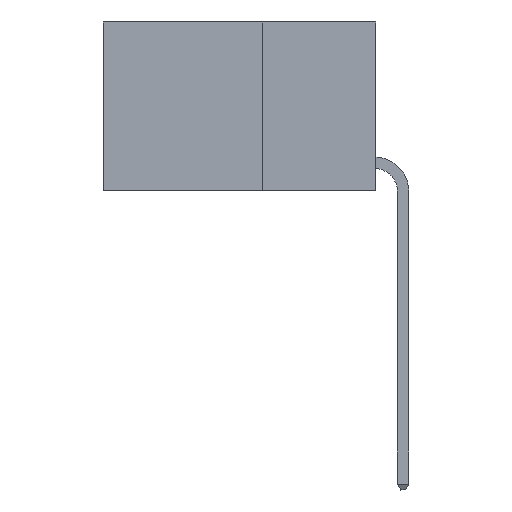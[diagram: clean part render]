
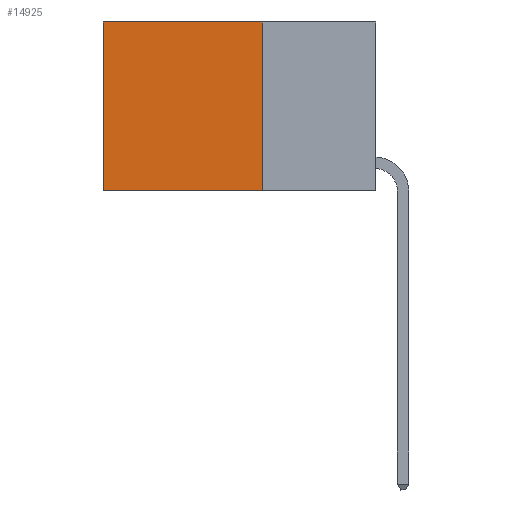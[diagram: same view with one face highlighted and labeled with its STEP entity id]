
A CAD part, left-side view. The second image highlights one B-rep face of the part: STEP entity #14925.
In plain terms, the highlighted planar face has unit normal (-1, 0, 0).
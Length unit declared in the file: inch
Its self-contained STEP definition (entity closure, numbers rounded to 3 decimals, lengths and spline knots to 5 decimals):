
#178 = EDGE_LOOP ( 'NONE', ( #12319, #1193, #4181, #5800 ) ) ;
#631 = FACE_OUTER_BOUND ( 'NONE', #178, .T. ) ;
#1193 = ORIENTED_EDGE ( 'NONE', *, *, #12555, .F. ) ;
#1260 = DIRECTION ( 'NONE',  ( 0., 0., -1. ) ) ;
#2142 = DIRECTION ( 'NONE',  ( 0., 1., 0. ) ) ;
#2449 = LINE ( 'NONE', #5815, #4506 ) ;
#2933 = VECTOR ( 'NONE', #1260, 39.37008 ) ;
#3328 = LINE ( 'NONE', #11789, #2933 ) ;
#3760 = DIRECTION ( 'NONE',  ( 0., 0., -1. ) ) ;
#4181 = ORIENTED_EDGE ( 'NONE', *, *, #6781, .F. ) ;
#4430 = EDGE_CURVE ( 'NONE', #8586, #11255, #3328, .T. ) ;
#4506 = VECTOR ( 'NONE', #7686, 39.37008 ) ;
#4978 = VERTEX_POINT ( 'NONE', #14207 ) ;
#5800 = ORIENTED_EDGE ( 'NONE', *, *, #12618, .T. ) ;
#5815 = CARTESIAN_POINT ( 'NONE',  ( 0.2625, 0.25, 0. ) ) ;
#5993 = CARTESIAN_POINT ( 'NONE',  ( 0.2625, 0.6, -0.37 ) ) ;
#6781 = EDGE_CURVE ( 'NONE', #4978, #9241, #12903, .T. ) ;
#6822 = CARTESIAN_POINT ( 'NONE',  ( 0.2625, 0.25, 0. ) ) ;
#7686 = DIRECTION ( 'NONE',  ( 0., 1., 0. ) ) ;
#7951 = DIRECTION ( 'NONE',  ( 0., 0., -1. ) ) ;
#8586 = VERTEX_POINT ( 'NONE', #13380 ) ;
#9241 = VERTEX_POINT ( 'NONE', #14566 ) ;
#9504 = VECTOR ( 'NONE', #3760, 39.37008 ) ;
#9573 = CARTESIAN_POINT ( 'NONE',  ( 0.2625, 0.25, 0. ) ) ;
#10325 = CARTESIAN_POINT ( 'NONE',  ( 0.2625, 0.25, -0.37 ) ) ;
#11032 = VECTOR ( 'NONE', #2142, 39.37008 ) ;
#11255 = VERTEX_POINT ( 'NONE', #5993 ) ;
#11789 = CARTESIAN_POINT ( 'NONE',  ( 0.2625, 0.6, 0. ) ) ;
#12319 = ORIENTED_EDGE ( 'NONE', *, *, #4430, .T. ) ;
#12516 = PLANE ( 'NONE',  #13845 ) ;
#12555 = EDGE_CURVE ( 'NONE', #9241, #11255, #13968, .T. ) ;
#12618 = EDGE_CURVE ( 'NONE', #4978, #8586, #2449, .T. ) ;
#12903 = LINE ( 'NONE', #9573, #9504 ) ;
#13380 = CARTESIAN_POINT ( 'NONE',  ( 0.2625, 0.6, 0. ) ) ;
#13845 = AXIS2_PLACEMENT_3D ( 'NONE', #6822, #14642, #7951 ) ;
#13968 = LINE ( 'NONE', #10325, #11032 ) ;
#14207 = CARTESIAN_POINT ( 'NONE',  ( 0.2625, 0.25, 0. ) ) ;
#14566 = CARTESIAN_POINT ( 'NONE',  ( 0.2625, 0.25, -0.37 ) ) ;
#14642 = DIRECTION ( 'NONE',  ( 1., 0., 0. ) ) ;
#14925 = ADVANCED_FACE ( 'NONE', ( #631 ), #12516, .F. ) ;
